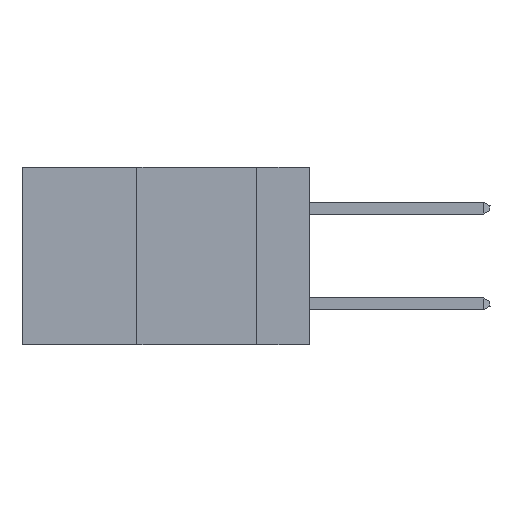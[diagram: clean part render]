
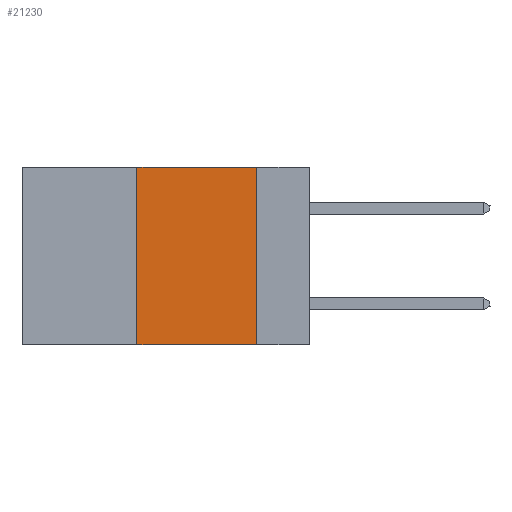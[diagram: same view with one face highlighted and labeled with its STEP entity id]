
A CAD part, left-side view. The second image highlights one B-rep face of the part: STEP entity #21230.
In plain terms, the highlighted planar face has unit normal (-1, 0, 0).
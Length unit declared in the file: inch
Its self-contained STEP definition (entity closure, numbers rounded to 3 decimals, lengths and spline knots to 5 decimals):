
#236 = EDGE_CURVE ( 'NONE', #1593, #14808, #7376, .T. ) ;
#1508 = VERTEX_POINT ( 'NONE', #19389 ) ;
#1593 = VERTEX_POINT ( 'NONE', #9384 ) ;
#1620 = EDGE_LOOP ( 'NONE', ( #8448, #13624, #16589, #21594 ) ) ;
#1638 = LINE ( 'NONE', #12912, #10156 ) ;
#1726 = DIRECTION ( 'NONE',  ( 0., -1., 0. ) ) ;
#1872 = VERTEX_POINT ( 'NONE', #19247 ) ;
#2539 = VECTOR ( 'NONE', #1726, 39.37008 ) ;
#4360 = CARTESIAN_POINT ( 'NONE',  ( 0., 0.6, 0. ) ) ;
#4382 = CARTESIAN_POINT ( 'NONE',  ( 0., 0.6, -0.37 ) ) ;
#6154 = CARTESIAN_POINT ( 'NONE',  ( 0., 0.11, 0. ) ) ;
#7376 = LINE ( 'NONE', #4382, #2539 ) ;
#7889 = DIRECTION ( 'NONE',  ( 0., 0., -1. ) ) ;
#8448 = ORIENTED_EDGE ( 'NONE', *, *, #9331, .F. ) ;
#8473 = EDGE_CURVE ( 'NONE', #1508, #1872, #1638, .T. ) ;
#9320 = FACE_OUTER_BOUND ( 'NONE', #1620, .T. ) ;
#9331 = EDGE_CURVE ( 'NONE', #1872, #14808, #17164, .T. ) ;
#9384 = CARTESIAN_POINT ( 'NONE',  ( 0., 0.36, -0.37 ) ) ;
#9494 = DIRECTION ( 'NONE',  ( 0., -1., 0. ) ) ;
#10156 = VECTOR ( 'NONE', #9494, 39.37008 ) ;
#11547 = DIRECTION ( 'NONE',  ( 0., 0., -1. ) ) ;
#12324 = LINE ( 'NONE', #18827, #16328 ) ;
#12912 = CARTESIAN_POINT ( 'NONE',  ( 0., 0.6, 0. ) ) ;
#13119 = VECTOR ( 'NONE', #7889, 39.37008 ) ;
#13624 = ORIENTED_EDGE ( 'NONE', *, *, #8473, .F. ) ;
#13826 = CARTESIAN_POINT ( 'NONE',  ( 0., 0.11, -0.37 ) ) ;
#14075 = EDGE_CURVE ( 'NONE', #1593, #1508, #12324, .T. ) ;
#14808 = VERTEX_POINT ( 'NONE', #13826 ) ;
#15338 = DIRECTION ( 'NONE',  ( 0., 0., 1. ) ) ;
#16328 = VECTOR ( 'NONE', #15338, 39.37008 ) ;
#16589 = ORIENTED_EDGE ( 'NONE', *, *, #14075, .F. ) ;
#16662 = PLANE ( 'NONE',  #22087 ) ;
#17164 = LINE ( 'NONE', #6154, #13119 ) ;
#18827 = CARTESIAN_POINT ( 'NONE',  ( 0., 0.36, 0. ) ) ;
#19247 = CARTESIAN_POINT ( 'NONE',  ( 0., 0.11, 0. ) ) ;
#19389 = CARTESIAN_POINT ( 'NONE',  ( 0., 0.36, 0. ) ) ;
#21230 = ADVANCED_FACE ( 'NONE', ( #9320 ), #16662, .F. ) ;
#21594 = ORIENTED_EDGE ( 'NONE', *, *, #236, .T. ) ;
#21730 = DIRECTION ( 'NONE',  ( 1., 0., 0. ) ) ;
#22087 = AXIS2_PLACEMENT_3D ( 'NONE', #4360, #21730, #11547 ) ;
